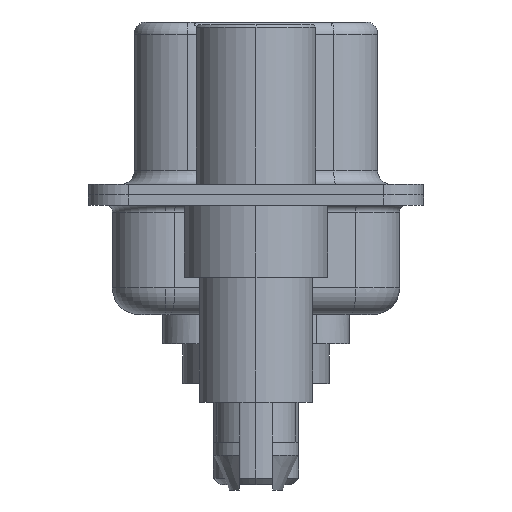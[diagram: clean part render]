
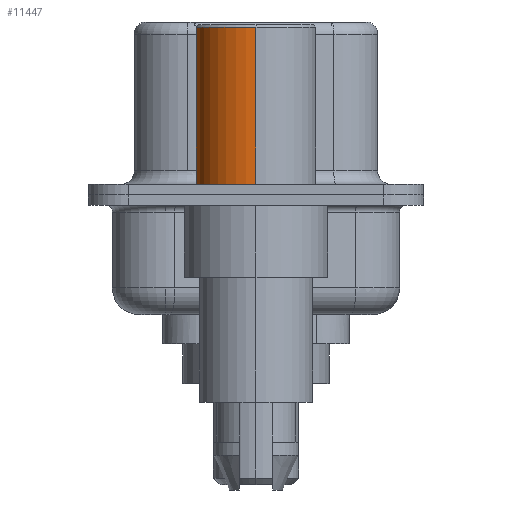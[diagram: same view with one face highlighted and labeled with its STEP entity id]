
A CAD part, left-side view. The second image highlights one B-rep face of the part: STEP entity #11447.
In plain terms, the highlighted cylindrical face has radius 2.25 mm (diameter 4.5 mm), a partial arc.
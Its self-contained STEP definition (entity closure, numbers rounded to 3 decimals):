
#926 = DIRECTION ( 'NONE',  ( 1., 0., 0. ) ) ;
#1280 = CYLINDRICAL_SURFACE ( 'NONE', #11324, 2.25 ) ;
#1787 = DIRECTION ( 'NONE',  ( 0., 0., 1. ) ) ;
#2413 = VERTEX_POINT ( 'NONE', #7814 ) ;
#2672 = VECTOR ( 'NONE', #4603, 1000. ) ;
#2835 = CARTESIAN_POINT ( 'NONE',  ( 2.25, 0., 0.581 ) ) ;
#3244 = CARTESIAN_POINT ( 'NONE',  ( 0., 0., 0.4 ) ) ;
#3526 = AXIS2_PLACEMENT_3D ( 'NONE', #3244, #1787, #12290 ) ;
#4149 = AXIS2_PLACEMENT_3D ( 'NONE', #12074, #12130, #11656 ) ;
#4478 = CARTESIAN_POINT ( 'NONE',  ( -2.25, 0., 6.3 ) ) ;
#4603 = DIRECTION ( 'NONE',  ( 0., 0., 1. ) ) ;
#5498 = LINE ( 'NONE', #12256, #2672 ) ;
#6569 = VECTOR ( 'NONE', #17637, 1000. ) ;
#7341 = CIRCLE ( 'NONE', #3526, 2.25 ) ;
#7512 = EDGE_CURVE ( 'NONE', #15462, #2413, #17887, .T. ) ;
#7769 = ORIENTED_EDGE ( 'NONE', *, *, #13003, .T. ) ;
#7814 = CARTESIAN_POINT ( 'NONE',  ( 2.25, 0., 6.3 ) ) ;
#8459 = CARTESIAN_POINT ( 'NONE',  ( 0., 0., 0.581 ) ) ;
#8560 = ORIENTED_EDGE ( 'NONE', *, *, #7512, .F. ) ;
#9019 = CIRCLE ( 'NONE', #4149, 2.25 ) ;
#10311 = VERTEX_POINT ( 'NONE', #4478 ) ;
#11324 = AXIS2_PLACEMENT_3D ( 'NONE', #8459, #19019, #926 ) ;
#11447 = ADVANCED_FACE ( 'NONE', ( #15414 ), #1280, .T. ) ;
#11656 = DIRECTION ( 'NONE',  ( 1., 0., 0. ) ) ;
#12074 = CARTESIAN_POINT ( 'NONE',  ( 0., 0., 6.3 ) ) ;
#12130 = DIRECTION ( 'NONE',  ( 0., 0., 1. ) ) ;
#12256 = CARTESIAN_POINT ( 'NONE',  ( -2.25, 0., 0.581 ) ) ;
#12290 = DIRECTION ( 'NONE',  ( 1., 0., 0. ) ) ;
#13003 = EDGE_CURVE ( 'NONE', #15462, #16187, #7341, .T. ) ;
#15414 = FACE_OUTER_BOUND ( 'NONE', #16702, .T. ) ;
#15462 = VERTEX_POINT ( 'NONE', #19361 ) ;
#15816 = ORIENTED_EDGE ( 'NONE', *, *, #19446, .F. ) ;
#16187 = VERTEX_POINT ( 'NONE', #17293 ) ;
#16702 = EDGE_LOOP ( 'NONE', ( #7769, #17602, #15816, #8560 ) ) ;
#17293 = CARTESIAN_POINT ( 'NONE',  ( -2.25, 0., 0.4 ) ) ;
#17602 = ORIENTED_EDGE ( 'NONE', *, *, #18905, .T. ) ;
#17637 = DIRECTION ( 'NONE',  ( 0., 0., 1. ) ) ;
#17887 = LINE ( 'NONE', #2835, #6569 ) ;
#18905 = EDGE_CURVE ( 'NONE', #16187, #10311, #5498, .T. ) ;
#19019 = DIRECTION ( 'NONE',  ( 0., 0., 1. ) ) ;
#19361 = CARTESIAN_POINT ( 'NONE',  ( 2.25, 0., 0.4 ) ) ;
#19446 = EDGE_CURVE ( 'NONE', #2413, #10311, #9019, .T. ) ;
